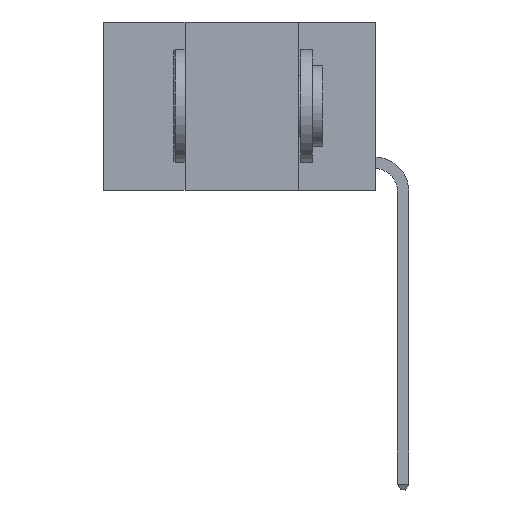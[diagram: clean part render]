
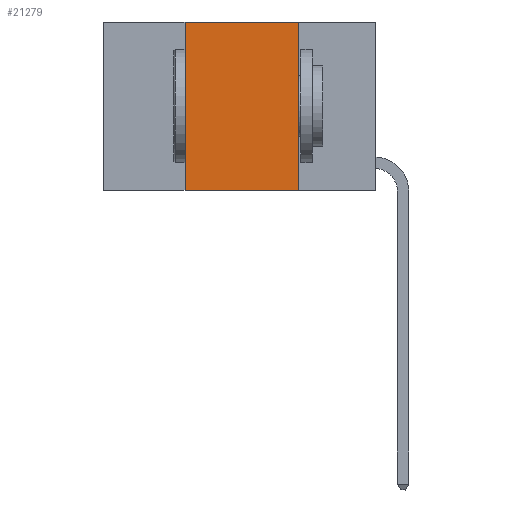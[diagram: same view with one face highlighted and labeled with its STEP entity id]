
A CAD part, left-side view. The second image highlights one B-rep face of the part: STEP entity #21279.
In plain terms, the highlighted planar face has unit normal (-1, 0, 0).
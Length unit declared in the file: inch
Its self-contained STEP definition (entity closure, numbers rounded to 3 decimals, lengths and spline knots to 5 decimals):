
#489 = VERTEX_POINT ( 'NONE', #23715 ) ;
#663 = FACE_OUTER_BOUND ( 'NONE', #3293, .T. ) ;
#2524 = CARTESIAN_POINT ( 'NONE',  ( 0., 0.42, 0. ) ) ;
#3154 = ORIENTED_EDGE ( 'NONE', *, *, #10369, .F. ) ;
#3293 = EDGE_LOOP ( 'NONE', ( #12334, #3154, #15085, #13193 ) ) ;
#3990 = LINE ( 'NONE', #18575, #7747 ) ;
#4912 = VECTOR ( 'NONE', #23719, 39.37008 ) ;
#4955 = DIRECTION ( 'NONE',  ( 1., 0., 0. ) ) ;
#5385 = EDGE_CURVE ( 'NONE', #11528, #489, #20081, .T. ) ;
#5685 = DIRECTION ( 'NONE',  ( 0., -1., 0. ) ) ;
#6837 = CARTESIAN_POINT ( 'NONE',  ( 0., 0.17, 0. ) ) ;
#7747 = VECTOR ( 'NONE', #18811, 39.37008 ) ;
#8594 = LINE ( 'NONE', #10309, #15903 ) ;
#9352 = EDGE_CURVE ( 'NONE', #18482, #489, #8594, .T. ) ;
#10309 = CARTESIAN_POINT ( 'NONE',  ( 0., 0.6, -0.37 ) ) ;
#10369 = EDGE_CURVE ( 'NONE', #21534, #11528, #14899, .T. ) ;
#11528 = VERTEX_POINT ( 'NONE', #13045 ) ;
#11664 = VECTOR ( 'NONE', #5685, 39.37008 ) ;
#12334 = ORIENTED_EDGE ( 'NONE', *, *, #5385, .F. ) ;
#12386 = EDGE_CURVE ( 'NONE', #18482, #21534, #3990, .T. ) ;
#13045 = CARTESIAN_POINT ( 'NONE',  ( 0., 0.17, 0. ) ) ;
#13193 = ORIENTED_EDGE ( 'NONE', *, *, #9352, .T. ) ;
#14206 = DIRECTION ( 'NONE',  ( 0., -1., 0. ) ) ;
#14403 = CARTESIAN_POINT ( 'NONE',  ( 0., 0.6, 0. ) ) ;
#14899 = LINE ( 'NONE', #19050, #11664 ) ;
#15085 = ORIENTED_EDGE ( 'NONE', *, *, #12386, .F. ) ;
#15297 = AXIS2_PLACEMENT_3D ( 'NONE', #14403, #4955, #21858 ) ;
#15903 = VECTOR ( 'NONE', #14206, 39.37008 ) ;
#17959 = PLANE ( 'NONE',  #15297 ) ;
#18482 = VERTEX_POINT ( 'NONE', #19659 ) ;
#18575 = CARTESIAN_POINT ( 'NONE',  ( 0., 0.42, 0. ) ) ;
#18811 = DIRECTION ( 'NONE',  ( 0., 0., 1. ) ) ;
#19050 = CARTESIAN_POINT ( 'NONE',  ( 0., 0.6, 0. ) ) ;
#19659 = CARTESIAN_POINT ( 'NONE',  ( 0., 0.42, -0.37 ) ) ;
#20081 = LINE ( 'NONE', #6837, #4912 ) ;
#21279 = ADVANCED_FACE ( 'NONE', ( #663 ), #17959, .F. ) ;
#21534 = VERTEX_POINT ( 'NONE', #2524 ) ;
#21858 = DIRECTION ( 'NONE',  ( 0., 0., -1. ) ) ;
#23715 = CARTESIAN_POINT ( 'NONE',  ( 0., 0.17, -0.37 ) ) ;
#23719 = DIRECTION ( 'NONE',  ( 0., 0., -1. ) ) ;
